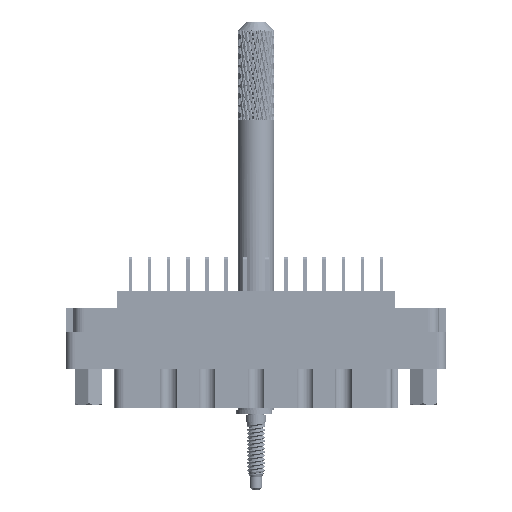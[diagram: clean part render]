
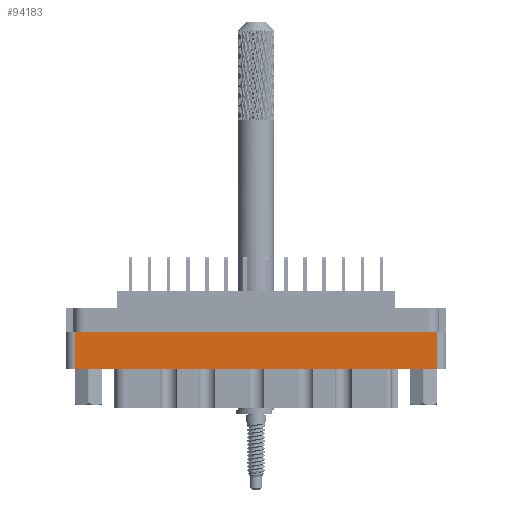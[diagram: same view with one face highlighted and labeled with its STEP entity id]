
A CAD part, front view. The second image highlights one B-rep face of the part: STEP entity #94183.
In plain terms, the highlighted planar face has unit normal (0, -1, 0).
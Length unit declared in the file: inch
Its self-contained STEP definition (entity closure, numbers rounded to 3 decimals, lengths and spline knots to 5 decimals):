
#1405 = EDGE_CURVE ( 'NONE', #44824, #32439, #118999, .T. ) ;
#3417 = VECTOR ( 'NONE', #58040, 39.37008 ) ;
#14126 = EDGE_CURVE ( 'NONE', #46701, #113092, #94169, .T. ) ;
#24099 = ORIENTED_EDGE ( 'NONE', *, *, #69213, .F. ) ;
#24549 = EDGE_LOOP ( 'NONE', ( #79819, #124659, #24099, #53203 ) ) ;
#24630 = DIRECTION ( 'NONE',  ( 0., 0., 1. ) ) ;
#27508 = CARTESIAN_POINT ( 'NONE',  ( 1.234, -0.438, -0.277 ) ) ;
#32439 = VERTEX_POINT ( 'NONE', #100428 ) ;
#38116 = PLANE ( 'NONE',  #99737 ) ;
#44824 = VERTEX_POINT ( 'NONE', #66204 ) ;
#46701 = VERTEX_POINT ( 'NONE', #105763 ) ;
#47475 = CARTESIAN_POINT ( 'NONE',  ( -1.296, -0.438, -0.798 ) ) ;
#50983 = EDGE_CURVE ( 'NONE', #44824, #113092, #87003, .T. ) ;
#52587 = LINE ( 'NONE', #67931, #116526 ) ;
#53203 = ORIENTED_EDGE ( 'NONE', *, *, #14126, .T. ) ;
#58040 = DIRECTION ( 'NONE',  ( 1., 0., 0. ) ) ;
#66183 = DIRECTION ( 'NONE',  ( 0., -1., 0. ) ) ;
#66204 = CARTESIAN_POINT ( 'NONE',  ( -1.234, -0.438, -0.277 ) ) ;
#67931 = CARTESIAN_POINT ( 'NONE',  ( 0., -0.438, -0.529 ) ) ;
#68246 = VECTOR ( 'NONE', #24630, 39.37008 ) ;
#69213 = EDGE_CURVE ( 'NONE', #46701, #32439, #52587, .T. ) ;
#79795 = CARTESIAN_POINT ( 'NONE',  ( 0., -0.438, -0.277 ) ) ;
#79819 = ORIENTED_EDGE ( 'NONE', *, *, #50983, .F. ) ;
#85516 = VECTOR ( 'NONE', #103863, 39.37008 ) ;
#87003 = LINE ( 'NONE', #79795, #3417 ) ;
#93534 = CARTESIAN_POINT ( 'NONE',  ( 1.234, -0.438, -0.798 ) ) ;
#94169 = LINE ( 'NONE', #93534, #68246 ) ;
#94183 = ADVANCED_FACE ( 'NONE', ( #112832 ), #38116, .T. ) ;
#99737 = AXIS2_PLACEMENT_3D ( 'NONE', #47475, #66183, #106175 ) ;
#100428 = CARTESIAN_POINT ( 'NONE',  ( -1.234, -0.438, -0.529 ) ) ;
#103863 = DIRECTION ( 'NONE',  ( 0., 0., -1. ) ) ;
#105763 = CARTESIAN_POINT ( 'NONE',  ( 1.234, -0.438, -0.529 ) ) ;
#106175 = DIRECTION ( 'NONE',  ( 0., 0., -1. ) ) ;
#106258 = DIRECTION ( 'NONE',  ( -1., 0., 0. ) ) ;
#112806 = CARTESIAN_POINT ( 'NONE',  ( -1.234, -0.438, -0.798 ) ) ;
#112832 = FACE_OUTER_BOUND ( 'NONE', #24549, .T. ) ;
#113092 = VERTEX_POINT ( 'NONE', #27508 ) ;
#116526 = VECTOR ( 'NONE', #106258, 39.37008 ) ;
#118999 = LINE ( 'NONE', #112806, #85516 ) ;
#124659 = ORIENTED_EDGE ( 'NONE', *, *, #1405, .T. ) ;
